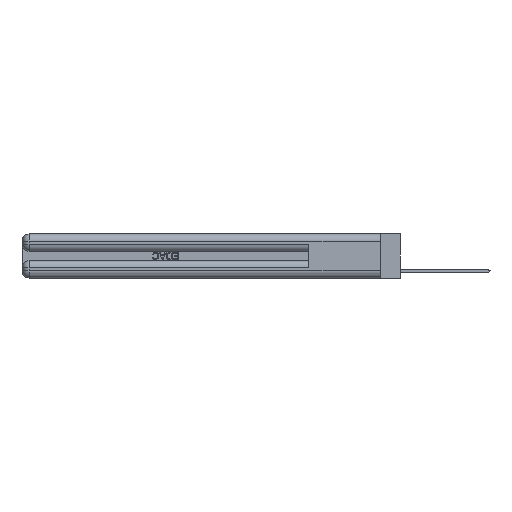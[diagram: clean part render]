
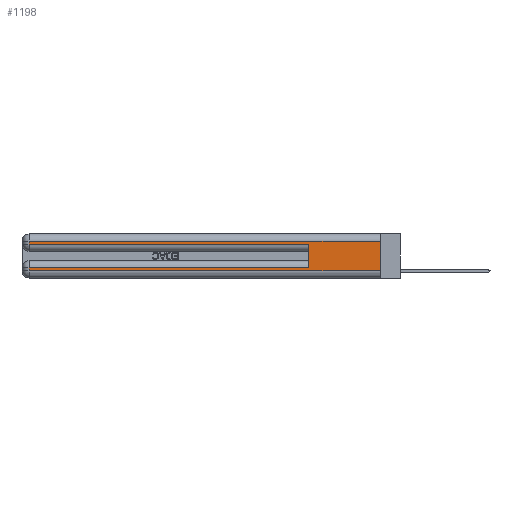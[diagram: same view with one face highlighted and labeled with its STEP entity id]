
A CAD part, left-side view. The second image highlights one B-rep face of the part: STEP entity #1198.
In plain terms, the highlighted planar face has unit normal (-1, 0, 0).
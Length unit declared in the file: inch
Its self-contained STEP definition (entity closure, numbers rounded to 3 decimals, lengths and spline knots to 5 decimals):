
#63 = EDGE_CURVE ( 'NONE', #34930, #28259, #20160, .T. ) ;
#1198 = ADVANCED_FACE ( 'NONE', ( #22184 ), #8625, .F. ) ;
#1528 = EDGE_LOOP ( 'NONE', ( #14938, #23868, #18132, #24037, #6239, #13031, #25924, #19483 ) ) ;
#2297 = DIRECTION ( 'NONE',  ( 1., 0., 0. ) ) ;
#2399 = LINE ( 'NONE', #13629, #17433 ) ;
#2697 = EDGE_CURVE ( 'NONE', #34930, #13419, #7030, .T. ) ;
#3020 = VECTOR ( 'NONE', #4623, 39.37008 ) ;
#3680 = VECTOR ( 'NONE', #19265, 39.37008 ) ;
#4623 = DIRECTION ( 'NONE',  ( 0., 0., 1. ) ) ;
#5016 = CARTESIAN_POINT ( 'NONE',  ( 0., 0., 0.37 ) ) ;
#5379 = CARTESIAN_POINT ( 'NONE',  ( 0., 0., 0.285 ) ) ;
#6239 = ORIENTED_EDGE ( 'NONE', *, *, #32386, .F. ) ;
#7030 = LINE ( 'NONE', #22932, #21626 ) ;
#7320 = EDGE_CURVE ( 'NONE', #11046, #30061, #2399, .T. ) ;
#8625 = PLANE ( 'NONE',  #20729 ) ;
#9324 = DIRECTION ( 'NONE',  ( 0., 0., -1. ) ) ;
#9383 = DIRECTION ( 'NONE',  ( 0., 1., 0. ) ) ;
#9792 = EDGE_CURVE ( 'NONE', #32831, #28259, #10424, .T. ) ;
#10424 = LINE ( 'NONE', #30105, #3680 ) ;
#10753 = CARTESIAN_POINT ( 'NONE',  ( 0., 0., 0.31 ) ) ;
#10935 = CARTESIAN_POINT ( 'NONE',  ( 0., 2.94, 0.285 ) ) ;
#11046 = VERTEX_POINT ( 'NONE', #31484 ) ;
#11666 = LINE ( 'NONE', #33684, #24822 ) ;
#12935 = LINE ( 'NONE', #21070, #3020 ) ;
#13031 = ORIENTED_EDGE ( 'NONE', *, *, #7320, .T. ) ;
#13419 = VERTEX_POINT ( 'NONE', #16058 ) ;
#13629 = CARTESIAN_POINT ( 'NONE',  ( 0., 0., 0.085 ) ) ;
#13638 = VECTOR ( 'NONE', #17613, 39.37008 ) ;
#14052 = EDGE_CURVE ( 'NONE', #30061, #32831, #28435, .T. ) ;
#14533 = CARTESIAN_POINT ( 'NONE',  ( 0., 2.94, 0.085 ) ) ;
#14763 = CARTESIAN_POINT ( 'NONE',  ( 0., 0., 0.37 ) ) ;
#14938 = ORIENTED_EDGE ( 'NONE', *, *, #63, .F. ) ;
#15219 = EDGE_CURVE ( 'NONE', #33816, #19840, #35372, .T. ) ;
#16002 = VECTOR ( 'NONE', #32650, 39.37008 ) ;
#16058 = CARTESIAN_POINT ( 'NONE',  ( 0., 2.94, 0.31 ) ) ;
#17433 = VECTOR ( 'NONE', #24279, 39.37008 ) ;
#17613 = DIRECTION ( 'NONE',  ( 0., 0., -1. ) ) ;
#18116 = CARTESIAN_POINT ( 'NONE',  ( 0., 0.6, 0.285 ) ) ;
#18132 = ORIENTED_EDGE ( 'NONE', *, *, #30804, .T. ) ;
#19265 = DIRECTION ( 'NONE',  ( 0., -1., 0. ) ) ;
#19483 = ORIENTED_EDGE ( 'NONE', *, *, #9792, .T. ) ;
#19840 = VERTEX_POINT ( 'NONE', #18116 ) ;
#20160 = LINE ( 'NONE', #14763, #30541 ) ;
#20729 = AXIS2_PLACEMENT_3D ( 'NONE', #5016, #2297, #35538 ) ;
#21070 = CARTESIAN_POINT ( 'NONE',  ( 0., 0.6, 0.145 ) ) ;
#21521 = CARTESIAN_POINT ( 'NONE',  ( 0., 2.94, 0.06 ) ) ;
#21626 = VECTOR ( 'NONE', #9383, 39.37008 ) ;
#22184 = FACE_OUTER_BOUND ( 'NONE', #1528, .T. ) ;
#22932 = CARTESIAN_POINT ( 'NONE',  ( 0., 0., 0.31 ) ) ;
#23380 = CARTESIAN_POINT ( 'NONE',  ( 0., 0., 0.06 ) ) ;
#23868 = ORIENTED_EDGE ( 'NONE', *, *, #2697, .T. ) ;
#24037 = ORIENTED_EDGE ( 'NONE', *, *, #15219, .T. ) ;
#24279 = DIRECTION ( 'NONE',  ( 0., 1., 0. ) ) ;
#24822 = VECTOR ( 'NONE', #32668, 39.37008 ) ;
#25924 = ORIENTED_EDGE ( 'NONE', *, *, #14052, .T. ) ;
#28259 = VERTEX_POINT ( 'NONE', #23380 ) ;
#28435 = LINE ( 'NONE', #30624, #13638 ) ;
#30061 = VERTEX_POINT ( 'NONE', #14533 ) ;
#30105 = CARTESIAN_POINT ( 'NONE',  ( 0., 0., 0.06 ) ) ;
#30541 = VECTOR ( 'NONE', #9324, 39.37008 ) ;
#30624 = CARTESIAN_POINT ( 'NONE',  ( 0., 2.94, 0.37 ) ) ;
#30804 = EDGE_CURVE ( 'NONE', #13419, #33816, #11666, .T. ) ;
#31484 = CARTESIAN_POINT ( 'NONE',  ( 0., 0.6, 0.085 ) ) ;
#32386 = EDGE_CURVE ( 'NONE', #11046, #19840, #12935, .T. ) ;
#32650 = DIRECTION ( 'NONE',  ( 0., -1., 0. ) ) ;
#32668 = DIRECTION ( 'NONE',  ( 0., 0., -1. ) ) ;
#32831 = VERTEX_POINT ( 'NONE', #21521 ) ;
#33684 = CARTESIAN_POINT ( 'NONE',  ( 0., 2.94, 0.37 ) ) ;
#33816 = VERTEX_POINT ( 'NONE', #10935 ) ;
#34930 = VERTEX_POINT ( 'NONE', #10753 ) ;
#35372 = LINE ( 'NONE', #5379, #16002 ) ;
#35538 = DIRECTION ( 'NONE',  ( 0., 0., -1. ) ) ;
